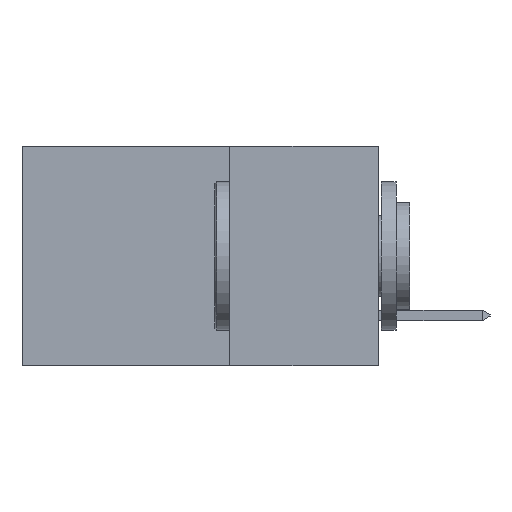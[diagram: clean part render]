
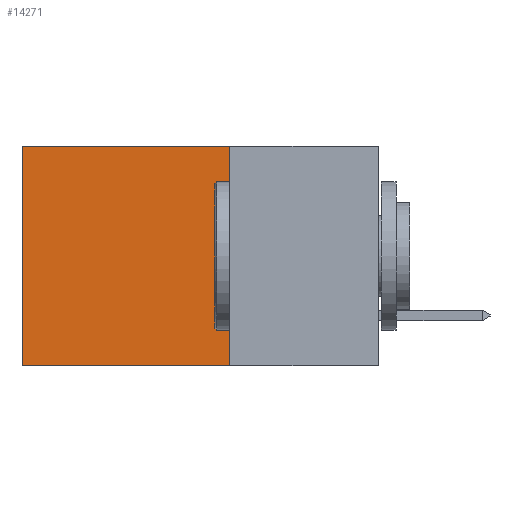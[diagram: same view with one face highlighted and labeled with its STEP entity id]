
A CAD part, left-side view. The second image highlights one B-rep face of the part: STEP entity #14271.
In plain terms, the highlighted planar face has unit normal (-1, 0, 0).
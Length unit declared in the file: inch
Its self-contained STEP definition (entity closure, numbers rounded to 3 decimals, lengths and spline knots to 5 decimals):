
#346 = CARTESIAN_POINT ( 'NONE',  ( 0.2615, 0.25, 0. ) ) ;
#865 = AXIS2_PLACEMENT_3D ( 'NONE', #12370, #2189, #14010 ) ;
#2120 = PLANE ( 'NONE',  #865 ) ;
#2189 = DIRECTION ( 'NONE',  ( 1., 0., 0. ) ) ;
#2489 = EDGE_CURVE ( 'NONE', #20092, #12322, #4605, .T. ) ;
#2753 = CARTESIAN_POINT ( 'NONE',  ( 0.2615, 0.6, -0.37 ) ) ;
#3524 = CARTESIAN_POINT ( 'NONE',  ( 0.2615, 0.6, -0.37 ) ) ;
#3812 = VECTOR ( 'NONE', #13850, 39.37008 ) ;
#4605 = LINE ( 'NONE', #13919, #17431 ) ;
#4737 = CARTESIAN_POINT ( 'NONE',  ( 0.2615, 0.6, 0. ) ) ;
#5737 = EDGE_CURVE ( 'NONE', #12322, #21580, #9206, .T. ) ;
#7995 = FACE_OUTER_BOUND ( 'NONE', #20293, .T. ) ;
#8594 = LINE ( 'NONE', #3524, #21225 ) ;
#9206 = LINE ( 'NONE', #10829, #17447 ) ;
#10692 = VERTEX_POINT ( 'NONE', #4737 ) ;
#10783 = DIRECTION ( 'NONE',  ( 0., 1., 0. ) ) ;
#10829 = CARTESIAN_POINT ( 'NONE',  ( 0.2615, 0.25, -0.37 ) ) ;
#12322 = VERTEX_POINT ( 'NONE', #17533 ) ;
#12370 = CARTESIAN_POINT ( 'NONE',  ( 0.2615, 0.25, -0.37 ) ) ;
#13395 = EDGE_CURVE ( 'NONE', #10692, #21580, #8594, .T. ) ;
#13759 = ORIENTED_EDGE ( 'NONE', *, *, #5737, .F. ) ;
#13850 = DIRECTION ( 'NONE',  ( 0., 1., 0. ) ) ;
#13919 = CARTESIAN_POINT ( 'NONE',  ( 0.2615, 0.25, -0.37 ) ) ;
#14010 = DIRECTION ( 'NONE',  ( 0., 0., -1. ) ) ;
#14271 = ADVANCED_FACE ( 'NONE', ( #7995 ), #2120, .F. ) ;
#14675 = DIRECTION ( 'NONE',  ( 0., 0., -1. ) ) ;
#16936 = DIRECTION ( 'NONE',  ( 0., 0., -1. ) ) ;
#17431 = VECTOR ( 'NONE', #14675, 39.37008 ) ;
#17447 = VECTOR ( 'NONE', #10783, 39.37008 ) ;
#17533 = CARTESIAN_POINT ( 'NONE',  ( 0.2615, 0.25, -0.37 ) ) ;
#17951 = EDGE_CURVE ( 'NONE', #20092, #10692, #21549, .T. ) ;
#17997 = ORIENTED_EDGE ( 'NONE', *, *, #2489, .F. ) ;
#18843 = CARTESIAN_POINT ( 'NONE',  ( 0.2615, 0.25, 0. ) ) ;
#20092 = VERTEX_POINT ( 'NONE', #18843 ) ;
#20293 = EDGE_LOOP ( 'NONE', ( #20576, #13759, #17997, #20424 ) ) ;
#20424 = ORIENTED_EDGE ( 'NONE', *, *, #17951, .T. ) ;
#20576 = ORIENTED_EDGE ( 'NONE', *, *, #13395, .T. ) ;
#21225 = VECTOR ( 'NONE', #16936, 39.37008 ) ;
#21549 = LINE ( 'NONE', #346, #3812 ) ;
#21580 = VERTEX_POINT ( 'NONE', #2753 ) ;
